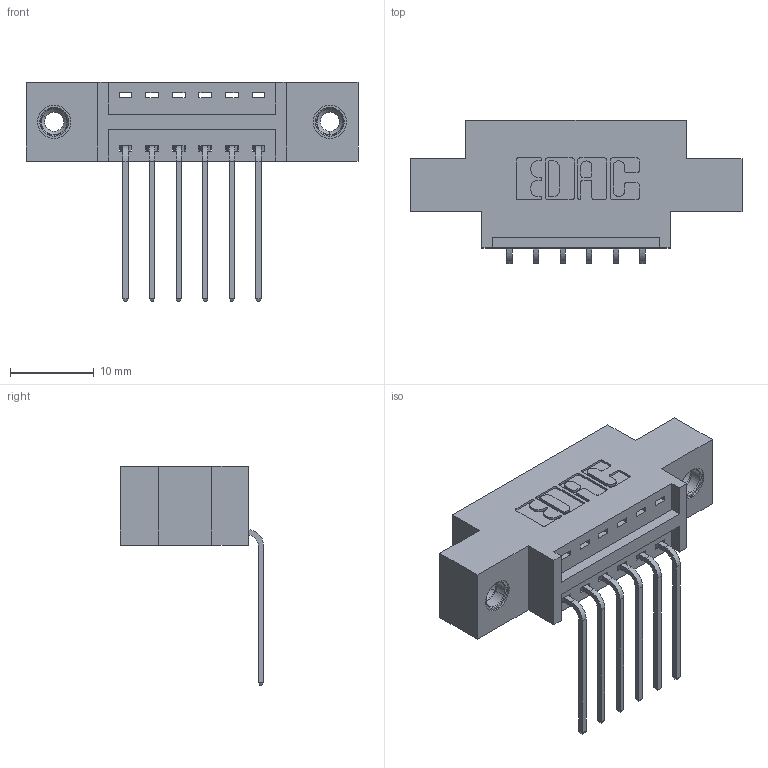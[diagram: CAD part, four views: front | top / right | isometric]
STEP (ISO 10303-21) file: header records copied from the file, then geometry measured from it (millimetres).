
FILE_DESCRIPTION (( 'STEP AP203' ), '1' );
FILE_NAME ('346-006-559-608.STEP', '2018-08-17T03:28:52', ( '' ), ( '' ), 'SwSTEP 2.0', 'SolidWorks 2016', '' );
FILE_SCHEMA (( 'CONFIG_CONTROL_DESIGN' ));
Length unit declared in the file: inch
Products named in the file (4): 346 Part_0.170 Offset - 0.156 Dia-TI; 345-292-001_558 559 Tail - 1; 345-250-001_345-250-003-102; 346-006-559-608
Assembly tree (9 placements, depth 2):
  346-006-559-608
    346 Part_0.170 Offset - 0.156 Dia-TI
    345-292-001_558 559 Tail - 1  x6
    345-250-001_345-250-003-102  x2
Bounding box: 39.62 x 17.08 x 26.16 mm (x, y, z)
Volume: 3403.7 mm3; surface area: 4167.1 mm2
Topology: 9 solids, 9 shells, 546 faces, 1569 edges, 1030 vertices
Faces by surface type: plane 364, cylinder 166, cone 12, torus 4
Entity records: 9972 total; most frequent: CARTESIAN_POINT 1705, ORIENTED_EDGE 1638, DIRECTION 1573, EDGE_CURVE 819, VECTOR 643, LINE 643, VERTEX_POINT 540, AXIS2_PLACEMENT_3D 465
